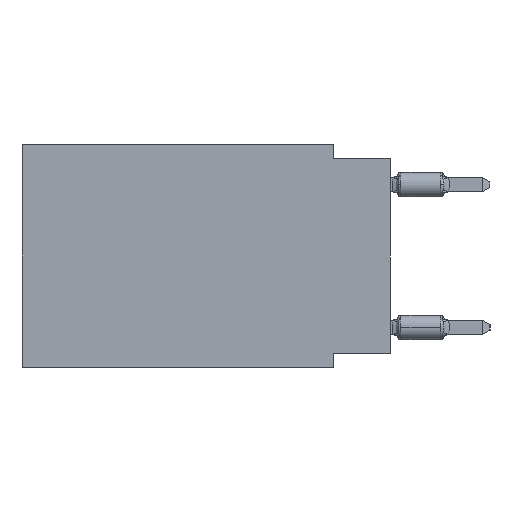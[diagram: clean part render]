
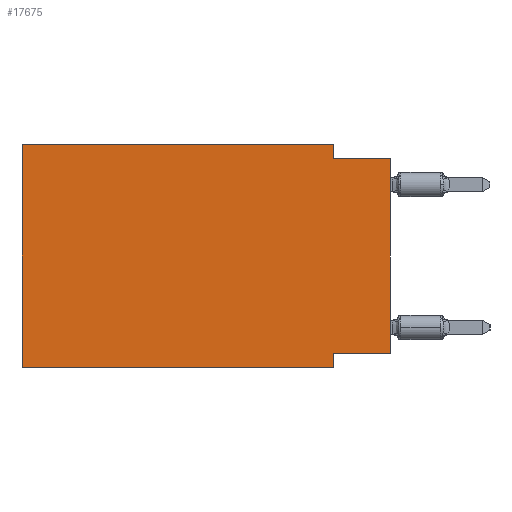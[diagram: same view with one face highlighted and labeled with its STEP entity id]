
A CAD part, left-side view. The second image highlights one B-rep face of the part: STEP entity #17675.
In plain terms, the highlighted planar face has unit normal (-1, 0, 0).
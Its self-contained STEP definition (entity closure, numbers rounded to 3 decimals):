
#2 = CARTESIAN_POINT ( 'NONE',  ( 0., 16.383, 0. ) ) ;
#380 = DIRECTION ( 'NONE',  ( 1., 0., 0. ) ) ;
#900 = EDGE_LOOP ( 'NONE', ( #6613, #7869, #4310, #16999, #13281, #20837, #20509, #30712 ) ) ;
#1634 = VERTEX_POINT ( 'NONE', #38578 ) ;
#2306 = EDGE_CURVE ( 'NONE', #38067, #38715, #14010, .T. ) ;
#2747 = VECTOR ( 'NONE', #4301, 1000. ) ;
#4034 = VECTOR ( 'NONE', #22594, 1000. ) ;
#4301 = DIRECTION ( 'NONE',  ( 0., 0., -1. ) ) ;
#4310 = ORIENTED_EDGE ( 'NONE', *, *, #33192, .F. ) ;
#4515 = CARTESIAN_POINT ( 'NONE',  ( 0., 2.54, -0.635 ) ) ;
#5810 = EDGE_CURVE ( 'NONE', #1634, #21064, #30242, .T. ) ;
#6198 = VECTOR ( 'NONE', #7996, 1000. ) ;
#6613 = ORIENTED_EDGE ( 'NONE', *, *, #26354, .T. ) ;
#6805 = CARTESIAN_POINT ( 'NONE',  ( 0., 0., -0.635 ) ) ;
#7649 = DIRECTION ( 'NONE',  ( 0., 0., 1. ) ) ;
#7704 = CARTESIAN_POINT ( 'NONE',  ( 0., 0., -9.271 ) ) ;
#7869 = ORIENTED_EDGE ( 'NONE', *, *, #2306, .F. ) ;
#7996 = DIRECTION ( 'NONE',  ( 0., -1., 0. ) ) ;
#9447 = CARTESIAN_POINT ( 'NONE',  ( 0., 2.54, 0. ) ) ;
#10217 = VECTOR ( 'NONE', #13803, 1000. ) ;
#10724 = DIRECTION ( 'NONE',  ( 0., 0., 1. ) ) ;
#10994 = CARTESIAN_POINT ( 'NONE',  ( 0., 0., -0.635 ) ) ;
#12010 = FACE_OUTER_BOUND ( 'NONE', #900, .T. ) ;
#12650 = DIRECTION ( 'NONE',  ( 0., 0., -1. ) ) ;
#12972 = VERTEX_POINT ( 'NONE', #34814 ) ;
#13281 = ORIENTED_EDGE ( 'NONE', *, *, #36358, .F. ) ;
#13590 = CARTESIAN_POINT ( 'NONE',  ( 0., 2.54, 0. ) ) ;
#13803 = DIRECTION ( 'NONE',  ( 0., -1., 0. ) ) ;
#14010 = LINE ( 'NONE', #10994, #6198 ) ;
#14395 = EDGE_CURVE ( 'NONE', #24466, #37439, #34612, .T. ) ;
#16532 = LINE ( 'NONE', #31935, #2747 ) ;
#16999 = ORIENTED_EDGE ( 'NONE', *, *, #5810, .F. ) ;
#17675 = ADVANCED_FACE ( 'NONE', ( #12010 ), #24234, .F. ) ;
#19871 = LINE ( 'NONE', #28882, #22049 ) ;
#20509 = ORIENTED_EDGE ( 'NONE', *, *, #29994, .F. ) ;
#20837 = ORIENTED_EDGE ( 'NONE', *, *, #14395, .T. ) ;
#21064 = VERTEX_POINT ( 'NONE', #13590 ) ;
#22049 = VECTOR ( 'NONE', #7649, 1000. ) ;
#22543 = CARTESIAN_POINT ( 'NONE',  ( 0., 0., 0. ) ) ;
#22594 = DIRECTION ( 'NONE',  ( 0., -1., 0. ) ) ;
#23577 = CARTESIAN_POINT ( 'NONE',  ( 0., 0., -9.271 ) ) ;
#24234 = PLANE ( 'NONE',  #27140 ) ;
#24466 = VERTEX_POINT ( 'NONE', #36870 ) ;
#26132 = EDGE_CURVE ( 'NONE', #26327, #12972, #26777, .T. ) ;
#26327 = VERTEX_POINT ( 'NONE', #7704 ) ;
#26354 = EDGE_CURVE ( 'NONE', #26327, #38715, #38351, .T. ) ;
#26775 = CARTESIAN_POINT ( 'NONE',  ( 0., 2.54, -9.906 ) ) ;
#26777 = LINE ( 'NONE', #23577, #35392 ) ;
#27140 = AXIS2_PLACEMENT_3D ( 'NONE', #27828, #380, #28036 ) ;
#27828 = CARTESIAN_POINT ( 'NONE',  ( 0., 16.383, 0. ) ) ;
#28036 = DIRECTION ( 'NONE',  ( 0., 0., -1. ) ) ;
#28882 = CARTESIAN_POINT ( 'NONE',  ( 0., 16.383, 0. ) ) ;
#29994 = EDGE_CURVE ( 'NONE', #12972, #37439, #16532, .T. ) ;
#30242 = LINE ( 'NONE', #2, #10217 ) ;
#30712 = ORIENTED_EDGE ( 'NONE', *, *, #26132, .F. ) ;
#31935 = CARTESIAN_POINT ( 'NONE',  ( 0., 2.54, -9.906 ) ) ;
#33192 = EDGE_CURVE ( 'NONE', #21064, #38067, #36473, .T. ) ;
#34231 = CARTESIAN_POINT ( 'NONE',  ( 0., 16.383, -9.906 ) ) ;
#34612 = LINE ( 'NONE', #34231, #4034 ) ;
#34806 = VECTOR ( 'NONE', #10724, 1000. ) ;
#34814 = CARTESIAN_POINT ( 'NONE',  ( 0., 2.54, -9.271 ) ) ;
#35392 = VECTOR ( 'NONE', #39389, 1000. ) ;
#35593 = VECTOR ( 'NONE', #12650, 1000. ) ;
#36358 = EDGE_CURVE ( 'NONE', #24466, #1634, #19871, .T. ) ;
#36473 = LINE ( 'NONE', #9447, #35593 ) ;
#36870 = CARTESIAN_POINT ( 'NONE',  ( 0., 16.383, -9.906 ) ) ;
#37439 = VERTEX_POINT ( 'NONE', #26775 ) ;
#38067 = VERTEX_POINT ( 'NONE', #4515 ) ;
#38351 = LINE ( 'NONE', #22543, #34806 ) ;
#38578 = CARTESIAN_POINT ( 'NONE',  ( 0., 16.383, 0. ) ) ;
#38715 = VERTEX_POINT ( 'NONE', #6805 ) ;
#39389 = DIRECTION ( 'NONE',  ( 0., 1., 0. ) ) ;
